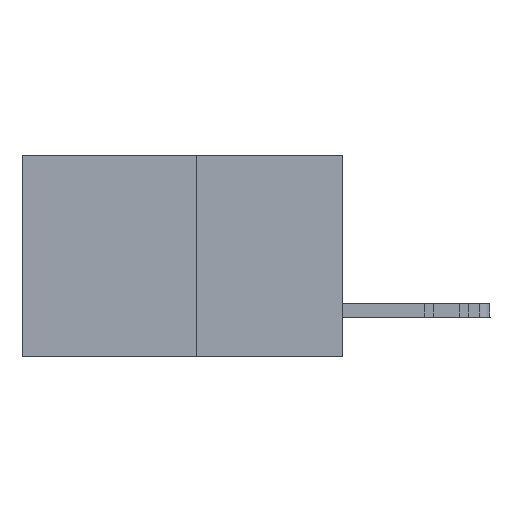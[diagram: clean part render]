
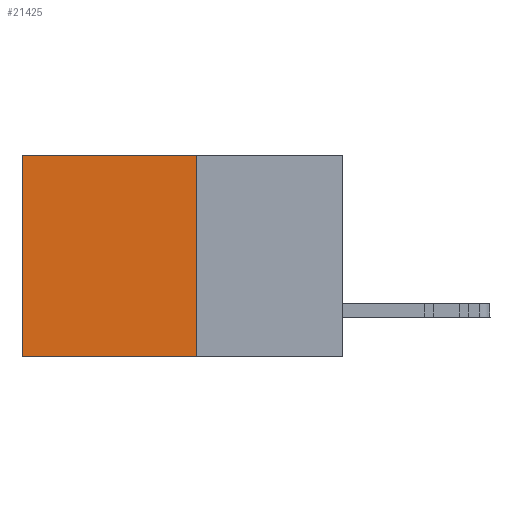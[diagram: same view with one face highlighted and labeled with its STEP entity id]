
A CAD part, left-side view. The second image highlights one B-rep face of the part: STEP entity #21425.
In plain terms, the highlighted planar face has unit normal (-1, 0, 0).
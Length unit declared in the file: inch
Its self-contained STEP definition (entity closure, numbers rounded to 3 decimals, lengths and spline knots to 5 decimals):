
#2062 = DIRECTION ( 'NONE',  ( 0., 1., 0. ) ) ;
#2666 = DIRECTION ( 'NONE',  ( 0., 0., -1. ) ) ;
#3140 = ORIENTED_EDGE ( 'NONE', *, *, #7171, .F. ) ;
#3803 = VERTEX_POINT ( 'NONE', #27940 ) ;
#4923 = DIRECTION ( 'NONE',  ( 0., 0., -1. ) ) ;
#5543 = PLANE ( 'NONE',  #6222 ) ;
#5695 = VECTOR ( 'NONE', #6146, 39.37008 ) ;
#6146 = DIRECTION ( 'NONE',  ( 0., 1., 0. ) ) ;
#6222 = AXIS2_PLACEMENT_3D ( 'NONE', #22415, #17621, #2666 ) ;
#6562 = ORIENTED_EDGE ( 'NONE', *, *, #19494, .T. ) ;
#7171 = EDGE_CURVE ( 'NONE', #24430, #3803, #26470, .T. ) ;
#9377 = EDGE_CURVE ( 'NONE', #26705, #24430, #26955, .T. ) ;
#9624 = DIRECTION ( 'NONE',  ( 0., 0., -1. ) ) ;
#12309 = VECTOR ( 'NONE', #9624, 39.37008 ) ;
#12674 = CARTESIAN_POINT ( 'NONE',  ( 0.277, 0.59, -0.37 ) ) ;
#14193 = EDGE_LOOP ( 'NONE', ( #6562, #3140, #19680, #26341 ) ) ;
#14936 = LINE ( 'NONE', #12674, #12309 ) ;
#15499 = VECTOR ( 'NONE', #4923, 39.37008 ) ;
#15526 = FACE_OUTER_BOUND ( 'NONE', #14193, .T. ) ;
#15704 = CARTESIAN_POINT ( 'NONE',  ( 0.277, 0.27, -0.37 ) ) ;
#17097 = CARTESIAN_POINT ( 'NONE',  ( 0.277, 0.27, 0. ) ) ;
#17621 = DIRECTION ( 'NONE',  ( 1., 0., 0. ) ) ;
#17878 = LINE ( 'NONE', #22701, #5695 ) ;
#19494 = EDGE_CURVE ( 'NONE', #26450, #3803, #14936, .T. ) ;
#19680 = ORIENTED_EDGE ( 'NONE', *, *, #9377, .F. ) ;
#21425 = ADVANCED_FACE ( 'NONE', ( #15526 ), #5543, .F. ) ;
#22128 = CARTESIAN_POINT ( 'NONE',  ( 0.277, 0.27, -0.37 ) ) ;
#22415 = CARTESIAN_POINT ( 'NONE',  ( 0.277, 0.27, -0.37 ) ) ;
#22701 = CARTESIAN_POINT ( 'NONE',  ( 0.277, 0.27, 0. ) ) ;
#23062 = CARTESIAN_POINT ( 'NONE',  ( 0.277, 0.59, 0. ) ) ;
#24430 = VERTEX_POINT ( 'NONE', #15704 ) ;
#25661 = VECTOR ( 'NONE', #2062, 39.37008 ) ;
#26341 = ORIENTED_EDGE ( 'NONE', *, *, #28390, .T. ) ;
#26450 = VERTEX_POINT ( 'NONE', #23062 ) ;
#26470 = LINE ( 'NONE', #22128, #25661 ) ;
#26705 = VERTEX_POINT ( 'NONE', #17097 ) ;
#26955 = LINE ( 'NONE', #28541, #15499 ) ;
#27940 = CARTESIAN_POINT ( 'NONE',  ( 0.277, 0.59, -0.37 ) ) ;
#28390 = EDGE_CURVE ( 'NONE', #26705, #26450, #17878, .T. ) ;
#28541 = CARTESIAN_POINT ( 'NONE',  ( 0.277, 0.27, -0.37 ) ) ;
